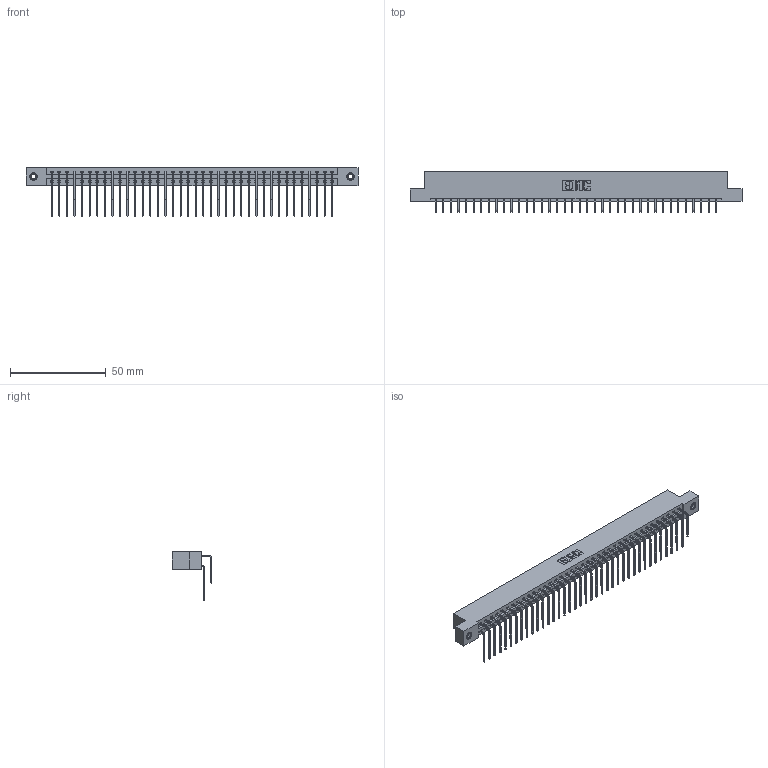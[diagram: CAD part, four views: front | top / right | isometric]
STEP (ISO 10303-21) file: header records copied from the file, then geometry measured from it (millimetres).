
FILE_DESCRIPTION (( 'STEP AP203' ), '1' );
FILE_NAME ('337-076-559-208.STEP', '2019-10-10T11:00:20', ( '' ), ( '' ), 'SwSTEP 2.0', 'SolidWorks 2016', '' );
FILE_SCHEMA (( 'CONFIG_CONTROL_DESIGN' ));
Length unit declared in the file: inch
Products named in the file (5): 345-292-001_559 Tail - 2; 337-076-559-208; 337 Part_Flush Mounting Lugs - 0.156 Dia-TI; 345-250-001_345-250-003-102; 345-292-001_558 559 Tail - 1
Assembly tree (79 placements, depth 2):
  337-076-559-208
    337 Part_Flush Mounting Lugs - 0.156 Dia-TI
    345-292-001_558 559 Tail - 1  x38
    345-292-001_559 Tail - 2  x38
    345-250-001_345-250-003-102  x2
Bounding box: 173.58 x 20.9 x 25.53 mm (x, y, z)
Volume: 18672.3 mm3; surface area: 23295.5 mm2
Topology: 79 solids, 79 shells, 4430 faces, 13139 edges, 8650 vertices
Faces by surface type: plane 3142, cylinder 1272, cone 12, torus 4
Entity records: 32950 total; most frequent: CARTESIAN_POINT 5580, ORIENTED_EDGE 5458, DIRECTION 4767, EDGE_CURVE 2729, VECTOR 2541, LINE 2541, VERTEX_POINT 1812, AXIS2_PLACEMENT_3D 1113
